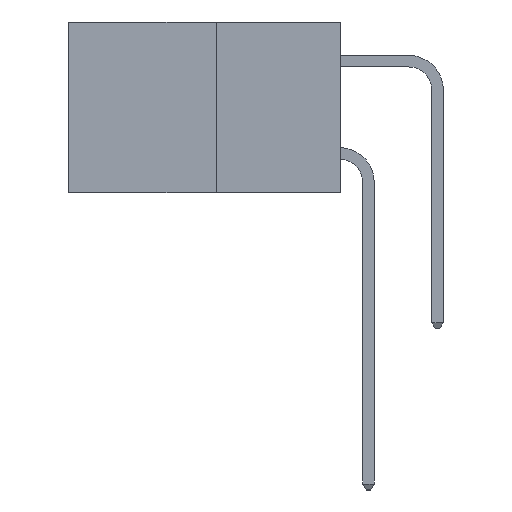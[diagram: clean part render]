
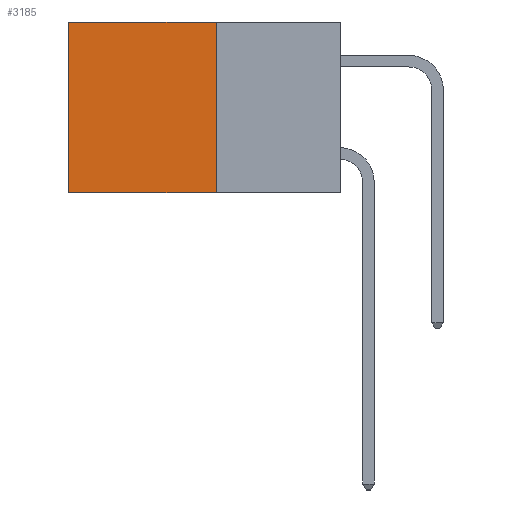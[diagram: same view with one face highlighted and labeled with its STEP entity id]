
A CAD part, left-side view. The second image highlights one B-rep face of the part: STEP entity #3185.
In plain terms, the highlighted planar face has unit normal (-1, 0, 0).
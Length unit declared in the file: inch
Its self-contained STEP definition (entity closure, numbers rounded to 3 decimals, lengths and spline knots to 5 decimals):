
#21 = DIRECTION ( 'NONE',  ( 0., 0., -1. ) ) ;
#1075 = EDGE_CURVE ( 'NONE', #3242, #1204, #8223, .T. ) ;
#1204 = VERTEX_POINT ( 'NONE', #1581 ) ;
#1453 = DIRECTION ( 'NONE',  ( 0., 0., -1. ) ) ;
#1581 = CARTESIAN_POINT ( 'NONE',  ( 0.277, 0.59, -0.37 ) ) ;
#2016 = EDGE_CURVE ( 'NONE', #9592, #3242, #6933, .T. ) ;
#2361 = CARTESIAN_POINT ( 'NONE',  ( 0.277, 0.27, -0.37 ) ) ;
#2655 = VECTOR ( 'NONE', #10199, 39.37008 ) ;
#2955 = EDGE_CURVE ( 'NONE', #9406, #1204, #7486, .T. ) ;
#3185 = ADVANCED_FACE ( 'NONE', ( #8581 ), #9317, .F. ) ;
#3242 = VERTEX_POINT ( 'NONE', #10381 ) ;
#4746 = DIRECTION ( 'NONE',  ( 0., 1., 0. ) ) ;
#4756 = CARTESIAN_POINT ( 'NONE',  ( 0.277, 0.27, 0. ) ) ;
#4799 = VECTOR ( 'NONE', #21, 39.37008 ) ;
#5122 = EDGE_CURVE ( 'NONE', #9592, #9406, #7051, .T. ) ;
#5791 = VECTOR ( 'NONE', #9639, 39.37008 ) ;
#6011 = ORIENTED_EDGE ( 'NONE', *, *, #2955, .T. ) ;
#6044 = ORIENTED_EDGE ( 'NONE', *, *, #2016, .F. ) ;
#6082 = ORIENTED_EDGE ( 'NONE', *, *, #5122, .T. ) ;
#6933 = LINE ( 'NONE', #7332, #4799 ) ;
#6945 = AXIS2_PLACEMENT_3D ( 'NONE', #2361, #9901, #1453 ) ;
#7051 = LINE ( 'NONE', #4756, #11390 ) ;
#7298 = EDGE_LOOP ( 'NONE', ( #6011, #8048, #6044, #6082 ) ) ;
#7332 = CARTESIAN_POINT ( 'NONE',  ( 0.277, 0.27, -0.37 ) ) ;
#7486 = LINE ( 'NONE', #10335, #2655 ) ;
#8048 = ORIENTED_EDGE ( 'NONE', *, *, #1075, .F. ) ;
#8223 = LINE ( 'NONE', #9517, #5791 ) ;
#8581 = FACE_OUTER_BOUND ( 'NONE', #7298, .T. ) ;
#9317 = PLANE ( 'NONE',  #6945 ) ;
#9406 = VERTEX_POINT ( 'NONE', #10664 ) ;
#9517 = CARTESIAN_POINT ( 'NONE',  ( 0.277, 0.27, -0.37 ) ) ;
#9592 = VERTEX_POINT ( 'NONE', #10152 ) ;
#9639 = DIRECTION ( 'NONE',  ( 0., 1., 0. ) ) ;
#9901 = DIRECTION ( 'NONE',  ( 1., 0., 0. ) ) ;
#10152 = CARTESIAN_POINT ( 'NONE',  ( 0.277, 0.27, 0. ) ) ;
#10199 = DIRECTION ( 'NONE',  ( 0., 0., -1. ) ) ;
#10335 = CARTESIAN_POINT ( 'NONE',  ( 0.277, 0.59, -0.37 ) ) ;
#10381 = CARTESIAN_POINT ( 'NONE',  ( 0.277, 0.27, -0.37 ) ) ;
#10664 = CARTESIAN_POINT ( 'NONE',  ( 0.277, 0.59, 0. ) ) ;
#11390 = VECTOR ( 'NONE', #4746, 39.37008 ) ;
